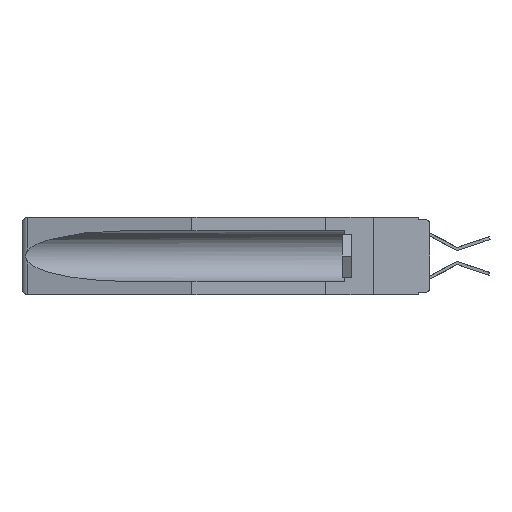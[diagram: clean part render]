
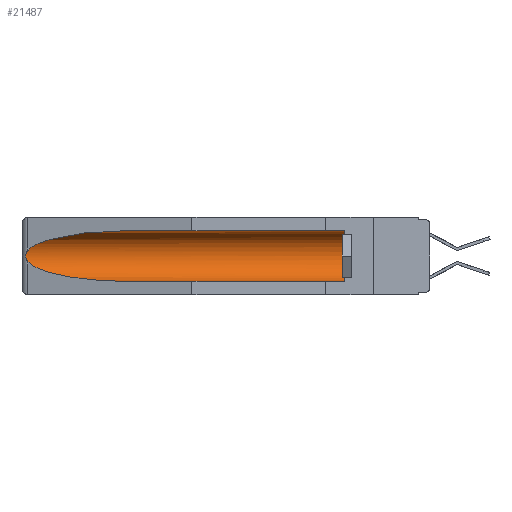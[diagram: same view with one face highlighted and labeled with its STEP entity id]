
A CAD part, left-side view. The second image highlights one B-rep face of the part: STEP entity #21487.
In plain terms, the highlighted cylindrical face has radius 2.857 mm (diameter 5.715 mm), a partial arc.
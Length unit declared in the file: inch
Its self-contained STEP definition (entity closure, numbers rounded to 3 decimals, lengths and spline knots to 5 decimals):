
#336 = DIRECTION ( 'NONE',  ( 0., 0., 1. ) ) ;
#670 = ORIENTED_EDGE ( 'NONE', *, *, #12075, .T. ) ;
#1315 = LINE ( 'NONE', #12288, #11639 ) ;
#1392 = CARTESIAN_POINT ( 'NONE',  ( 0.26537, 1.52718, -0.14972 ) ) ;
#2077 = CARTESIAN_POINT ( 'NONE',  ( 0.26537, 1.52718, -0.14972 ) ) ;
#2210 = CARTESIAN_POINT ( 'NONE',  ( 0.155, 1.07973, -0.284 ) ) ;
#2238 = CYLINDRICAL_SURFACE ( 'NONE', #14619, 0.1125 ) ;
#2319 = CARTESIAN_POINT ( 'NONE',  ( 0.26537, 1.52718, -0.19328 ) ) ;
#2519 = VERTEX_POINT ( 'NONE', #2706 ) ;
#2562 = EDGE_CURVE ( 'NONE', #9024, #9253, #20333, .T. ) ;
#2695 = VERTEX_POINT ( 'NONE', #2210 ) ;
#2706 = CARTESIAN_POINT ( 'NONE',  ( 0.155, 1.07973, -0.059 ) ) ;
#3050 = CARTESIAN_POINT ( 'NONE',  ( 0.155, 0.126, -0.059 ) ) ;
#3069 = CARTESIAN_POINT ( 'NONE',  ( 0.2675, 1.53308, -0.17534 ) ) ;
#4620 = EDGE_CURVE ( 'NONE', #5619, #2695, #21529, .T. ) ;
#4865 = CARTESIAN_POINT ( 'NONE',  ( 0.26654, 1.53092, -0.15636 ) ) ;
#5100 = CARTESIAN_POINT ( 'NONE',  ( 0.26537, 1.52718, -0.19328 ) ) ;
#5240 = DIRECTION ( 'NONE',  ( 0., 1., 0. ) ) ;
#5451 = CARTESIAN_POINT ( 'NONE',  ( 0.155, 0.126, -0.284 ) ) ;
#5619 = VERTEX_POINT ( 'NONE', #2319 ) ;
#5855 = CARTESIAN_POINT ( 'NONE',  ( 0.26537, 1.52718, -0.14972 ) ) ;
#6195 = EDGE_CURVE ( 'NONE', #16683, #5619, #22630, .T. ) ;
#6239 = ORIENTED_EDGE ( 'NONE', *, *, #2562, .T. ) ;
#6465 = CARTESIAN_POINT ( 'NONE',  ( 0.155, 1.07973, -0.284 ) ) ;
#6863 = DIRECTION ( 'NONE',  ( 0., 0., 1. ) ) ;
#6979 = CARTESIAN_POINT ( 'NONE',  ( 0.155, 0.126, -0.1715 ) ) ;
#7715 = CARTESIAN_POINT ( 'NONE',  ( 0.155, -0.30754, -0.1715 ) ) ;
#8292 = ORIENTED_EDGE ( 'NONE', *, *, #22392, .T. ) ;
#8668 = CARTESIAN_POINT ( 'NONE',  ( 0.2673, 1.5327, -0.16383 ) ) ;
#8895 = CARTESIAN_POINT ( 'NONE',  ( 0.26655, 1.53094, -0.18657 ) ) ;
#9024 = VERTEX_POINT ( 'NONE', #5451 ) ;
#9253 = VERTEX_POINT ( 'NONE', #3050 ) ;
#9780 = CARTESIAN_POINT ( 'NONE',  ( 0.21114, 1.30732, -0.059 ) ) ;
#10340 = CARTESIAN_POINT ( 'NONE',  ( 0.26597, 1.5296, -0.19026 ) ) ;
#11639 = VECTOR ( 'NONE', #15737, 39.37008 ) ;
#11653 = VECTOR ( 'NONE', #5240, 39.37008 ) ;
#12015 = CARTESIAN_POINT ( 'NONE',  ( 0.2675, 1.53308, -0.16763 ) ) ;
#12075 = EDGE_CURVE ( 'NONE', #2519, #16683, #20152, .T. ) ;
#12288 = CARTESIAN_POINT ( 'NONE',  ( 0.155, -0.30754, -0.059 ) ) ;
#13234 = CARTESIAN_POINT ( 'NONE',  ( 0.25451, 1.48313, -0.09465 ) ) ;
#13789 = ORIENTED_EDGE ( 'NONE', *, *, #22811, .F. ) ;
#14619 = AXIS2_PLACEMENT_3D ( 'NONE', #7715, #16646, #336 ) ;
#15737 = DIRECTION ( 'NONE',  ( 0., 1., 0. ) ) ;
#15945 = CARTESIAN_POINT ( 'NONE',  ( 0.155, -0.30754, -0.284 ) ) ;
#16283 = EDGE_LOOP ( 'NONE', ( #670, #19387, #17002, #13789, #6239, #8292 ) ) ;
#16407 = FACE_OUTER_BOUND ( 'NONE', #16283, .T. ) ;
#16646 = DIRECTION ( 'NONE',  ( 0., 1., 0. ) ) ;
#16683 = VERTEX_POINT ( 'NONE', #2077 ) ;
#16795 = CARTESIAN_POINT ( 'NONE',  ( 0.155, 1.07973, -0.059 ) ) ;
#17002 = ORIENTED_EDGE ( 'NONE', *, *, #4620, .T. ) ;
#18971 = CARTESIAN_POINT ( 'NONE',  ( 0.25451, 1.48313, -0.24835 ) ) ;
#19189 = AXIS2_PLACEMENT_3D ( 'NONE', #6979, #23162, #6863 ) ;
#19387 = ORIENTED_EDGE ( 'NONE', *, *, #6195, .T. ) ;
#19606 = CARTESIAN_POINT ( 'NONE',  ( 0.26597, 1.52961, -0.15275 ) ) ;
#20152 =( BOUNDED_CURVE ( )  B_SPLINE_CURVE ( 3, ( #16795, #9780, #13234, #5855 ),
 .UNSPECIFIED., .F., .F. ) 
 B_SPLINE_CURVE_WITH_KNOTS ( ( 4, 4 ),
 ( 4.71239, 6.08839 ),
 .UNSPECIFIED. ) 
 CURVE ( )  GEOMETRIC_REPRESENTATION_ITEM ( )  RATIONAL_B_SPLINE_CURVE ( ( 1., 0.848, 0.848, 1. ) ) 
 REPRESENTATION_ITEM ( '' )  );
#20333 = CIRCLE ( 'NONE', #19189, 0.1125 ) ;
#20624 = CARTESIAN_POINT ( 'NONE',  ( 0.26537, 1.52718, -0.19328 ) ) ;
#21022 = CARTESIAN_POINT ( 'NONE',  ( 0.2673, 1.53269, -0.17917 ) ) ;
#21487 = ADVANCED_FACE ( 'NONE', ( #16407 ), #2238, .F. ) ;
#21501 = LINE ( 'NONE', #15945, #11653 ) ;
#21529 =( BOUNDED_CURVE ( )  B_SPLINE_CURVE ( 3, ( #20624, #18971, #22757, #6465 ),
 .UNSPECIFIED., .F., .F. ) 
 B_SPLINE_CURVE_WITH_KNOTS ( ( 4, 4 ),
 ( 0.1948, 1.5708 ),
 .UNSPECIFIED. ) 
 CURVE ( )  GEOMETRIC_REPRESENTATION_ITEM ( )  RATIONAL_B_SPLINE_CURVE ( ( 1., 0.848, 0.848, 1. ) ) 
 REPRESENTATION_ITEM ( '' )  );
#22392 = EDGE_CURVE ( 'NONE', #9253, #2519, #1315, .T. ) ;
#22630 = B_SPLINE_CURVE_WITH_KNOTS ( 'NONE', 3,
 ( #1392, #19606, #4865, #8668, #12015, #3069, #21022, #8895, #10340, #5100 ),
 .UNSPECIFIED., .F., .F.,
 ( 4, 2, 2, 2, 4 ),
 ( 0., 0.00029, 0.00058, 0.00087, 0.00117 ),
 .UNSPECIFIED. ) ;
#22757 = CARTESIAN_POINT ( 'NONE',  ( 0.21114, 1.30732, -0.284 ) ) ;
#22811 = EDGE_CURVE ( 'NONE', #9024, #2695, #21501, .T. ) ;
#23162 = DIRECTION ( 'NONE',  ( 0., -1., 0. ) ) ;
